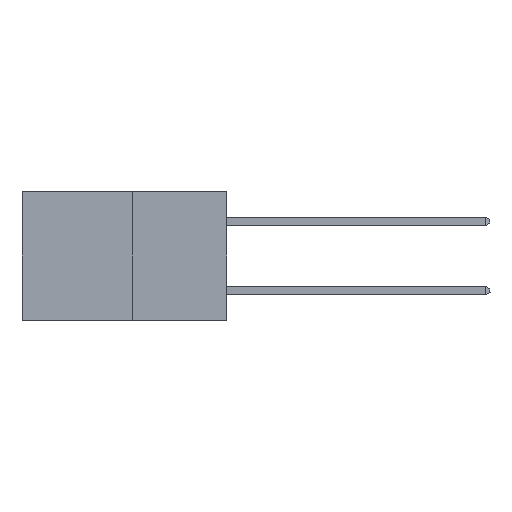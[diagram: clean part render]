
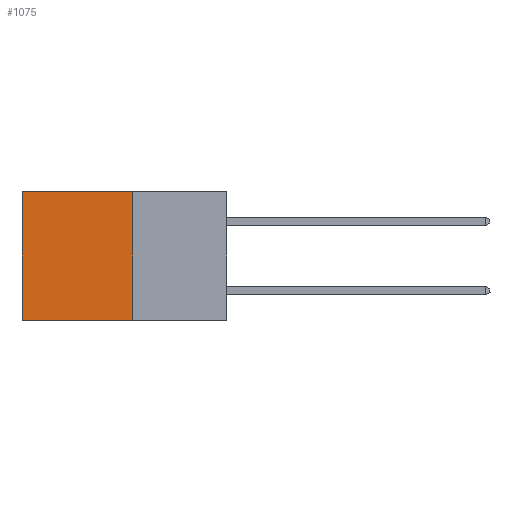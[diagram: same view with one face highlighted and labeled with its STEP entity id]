
A CAD part, left-side view. The second image highlights one B-rep face of the part: STEP entity #1075.
In plain terms, the highlighted planar face has unit normal (-1, 0, 0).
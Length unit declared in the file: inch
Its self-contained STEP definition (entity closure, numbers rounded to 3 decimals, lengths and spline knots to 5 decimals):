
#616 = CARTESIAN_POINT ( 'NONE',  ( 0.277, 0.59, 0. ) ) ;
#722 = VECTOR ( 'NONE', #8840, 39.37008 ) ;
#1075 = ADVANCED_FACE ( 'NONE', ( #3026 ), #15750, .F. ) ;
#2140 = CARTESIAN_POINT ( 'NONE',  ( 0.277, 0.59, -0.37 ) ) ;
#3026 = FACE_OUTER_BOUND ( 'NONE', #6959, .T. ) ;
#3366 = LINE ( 'NONE', #8121, #6578 ) ;
#4034 = ORIENTED_EDGE ( 'NONE', *, *, #7490, .F. ) ;
#4358 = CARTESIAN_POINT ( 'NONE',  ( 0.277, 0.27, -0.37 ) ) ;
#4359 = LINE ( 'NONE', #15669, #7969 ) ;
#4937 = ORIENTED_EDGE ( 'NONE', *, *, #16121, .F. ) ;
#4977 = LINE ( 'NONE', #9164, #8151 ) ;
#5007 = VERTEX_POINT ( 'NONE', #616 ) ;
#5702 = EDGE_CURVE ( 'NONE', #6015, #5007, #4359, .T. ) ;
#6015 = VERTEX_POINT ( 'NONE', #12914 ) ;
#6364 = EDGE_CURVE ( 'NONE', #5007, #12758, #4977, .T. ) ;
#6578 = VECTOR ( 'NONE', #7717, 39.37008 ) ;
#6959 = EDGE_LOOP ( 'NONE', ( #9579, #4034, #4937, #17094 ) ) ;
#7490 = EDGE_CURVE ( 'NONE', #11286, #12758, #3366, .T. ) ;
#7717 = DIRECTION ( 'NONE',  ( 0., 1., 0. ) ) ;
#7969 = VECTOR ( 'NONE', #15631, 39.37008 ) ;
#8121 = CARTESIAN_POINT ( 'NONE',  ( 0.277, 0.27, -0.37 ) ) ;
#8151 = VECTOR ( 'NONE', #8812, 39.37008 ) ;
#8520 = AXIS2_PLACEMENT_3D ( 'NONE', #14238, #16226, #14006 ) ;
#8812 = DIRECTION ( 'NONE',  ( 0., 0., -1. ) ) ;
#8840 = DIRECTION ( 'NONE',  ( 0., 0., -1. ) ) ;
#9164 = CARTESIAN_POINT ( 'NONE',  ( 0.277, 0.59, -0.37 ) ) ;
#9579 = ORIENTED_EDGE ( 'NONE', *, *, #6364, .T. ) ;
#11286 = VERTEX_POINT ( 'NONE', #4358 ) ;
#12046 = LINE ( 'NONE', #15657, #722 ) ;
#12758 = VERTEX_POINT ( 'NONE', #2140 ) ;
#12914 = CARTESIAN_POINT ( 'NONE',  ( 0.277, 0.27, 0. ) ) ;
#14006 = DIRECTION ( 'NONE',  ( 0., 0., -1. ) ) ;
#14238 = CARTESIAN_POINT ( 'NONE',  ( 0.277, 0.27, -0.37 ) ) ;
#15631 = DIRECTION ( 'NONE',  ( 0., 1., 0. ) ) ;
#15657 = CARTESIAN_POINT ( 'NONE',  ( 0.277, 0.27, -0.37 ) ) ;
#15669 = CARTESIAN_POINT ( 'NONE',  ( 0.277, 0.27, 0. ) ) ;
#15750 = PLANE ( 'NONE',  #8520 ) ;
#16121 = EDGE_CURVE ( 'NONE', #6015, #11286, #12046, .T. ) ;
#16226 = DIRECTION ( 'NONE',  ( 1., 0., 0. ) ) ;
#17094 = ORIENTED_EDGE ( 'NONE', *, *, #5702, .T. ) ;
